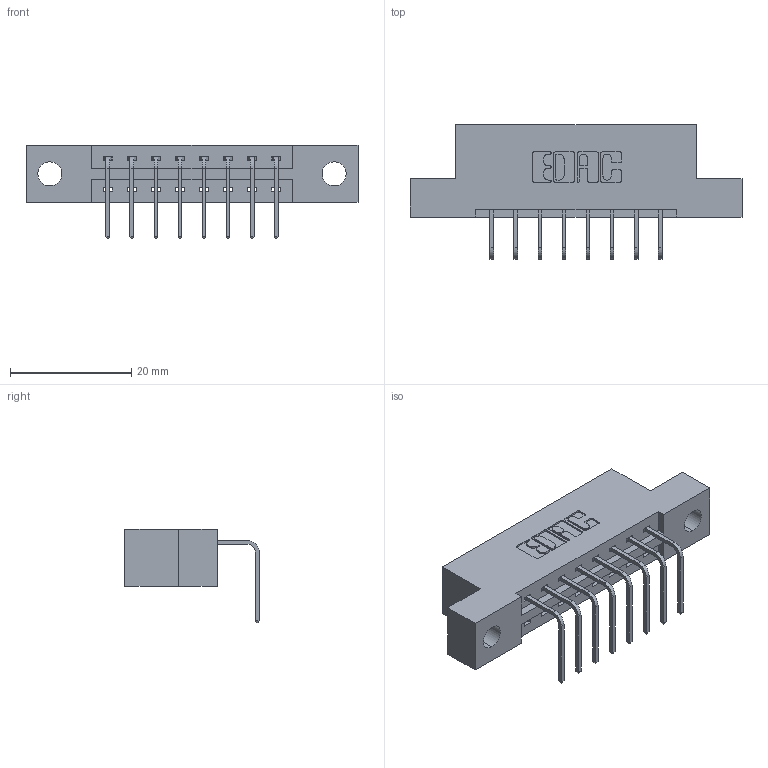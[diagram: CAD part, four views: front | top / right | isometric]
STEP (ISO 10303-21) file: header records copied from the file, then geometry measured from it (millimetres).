
FILE_DESCRIPTION (( 'STEP AP203' ), '1' );
FILE_NAME ('387-008-558-104.STEP', '2019-10-07T15:55:48', ( '' ), ( '' ), 'SwSTEP 2.0', 'SolidWorks 2016', '' );
FILE_SCHEMA (( 'CONFIG_CONTROL_DESIGN' ));
Length unit declared in the file: inch
Products named in the file (3): 345-292-001_558 Tail - 2; 387-008-558-104; 337 Part_Flush Mounting Lugs - 0.156 Dia-TH
Assembly tree (9 placements, depth 2):
  387-008-558-104
    337 Part_Flush Mounting Lugs - 0.156 Dia-TH
    345-292-001_558 Tail - 2  x8
Bounding box: 54.71 x 22.17 x 15.37 mm (x, y, z)
Volume: 5199.7 mm3; surface area: 5143.4 mm2
Topology: 9 solids, 9 shells, 626 faces, 1863 edges, 1230 vertices
Faces by surface type: plane 454, cylinder 172
Entity records: 10431 total; most frequent: CARTESIAN_POINT 1822, ORIENTED_EDGE 1766, DIRECTION 1603, EDGE_CURVE 883, VECTOR 755, LINE 755, VERTEX_POINT 586, AXIS2_PLACEMENT_3D 424
